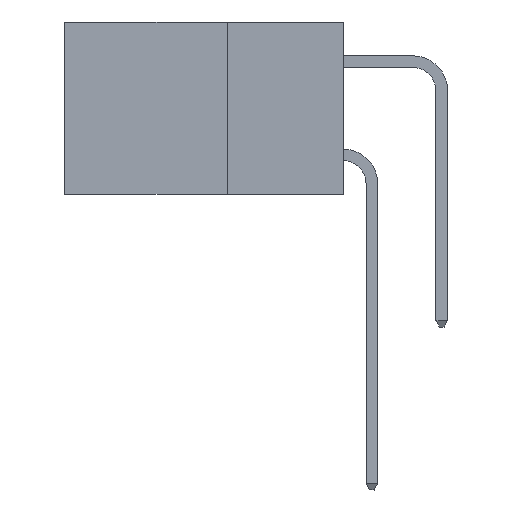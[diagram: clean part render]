
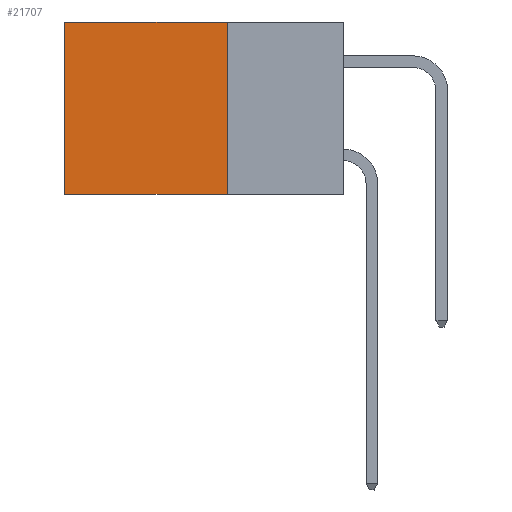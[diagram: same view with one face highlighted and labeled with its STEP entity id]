
A CAD part, left-side view. The second image highlights one B-rep face of the part: STEP entity #21707.
In plain terms, the highlighted planar face has unit normal (-1, 0, 0).
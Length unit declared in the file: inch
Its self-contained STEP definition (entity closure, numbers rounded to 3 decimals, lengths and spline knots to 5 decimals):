
#873 = LINE ( 'NONE', #14879, #6873 ) ;
#923 = ORIENTED_EDGE ( 'NONE', *, *, #19114, .T. ) ;
#928 = CARTESIAN_POINT ( 'NONE',  ( 0.2615, 0.25, -0.37 ) ) ;
#1483 = CARTESIAN_POINT ( 'NONE',  ( 0.2615, 0.25, 0. ) ) ;
#2189 = CARTESIAN_POINT ( 'NONE',  ( 0.2615, 0.25, -0.37 ) ) ;
#2313 = AXIS2_PLACEMENT_3D ( 'NONE', #5311, #12302, #3360 ) ;
#2867 = VECTOR ( 'NONE', #5848, 39.37008 ) ;
#2991 = VERTEX_POINT ( 'NONE', #1483 ) ;
#3360 = DIRECTION ( 'NONE',  ( 0., 0., -1. ) ) ;
#3834 = ORIENTED_EDGE ( 'NONE', *, *, #14002, .T. ) ;
#3910 = LINE ( 'NONE', #2189, #2867 ) ;
#4066 = VECTOR ( 'NONE', #19971, 39.37008 ) ;
#4170 = LINE ( 'NONE', #14845, #10130 ) ;
#4768 = ORIENTED_EDGE ( 'NONE', *, *, #12887, .F. ) ;
#5311 = CARTESIAN_POINT ( 'NONE',  ( 0.2615, 0.25, -0.37 ) ) ;
#5848 = DIRECTION ( 'NONE',  ( 0., 1., 0. ) ) ;
#6873 = VECTOR ( 'NONE', #21893, 39.37008 ) ;
#6913 = FACE_OUTER_BOUND ( 'NONE', #11136, .T. ) ;
#10130 = VECTOR ( 'NONE', #16350, 39.37008 ) ;
#11136 = EDGE_LOOP ( 'NONE', ( #923, #19903, #4768, #3834 ) ) ;
#11342 = CARTESIAN_POINT ( 'NONE',  ( 0.2615, 0.6, -0.37 ) ) ;
#11467 = LINE ( 'NONE', #11342, #4066 ) ;
#12302 = DIRECTION ( 'NONE',  ( 1., 0., 0. ) ) ;
#12887 = EDGE_CURVE ( 'NONE', #2991, #14870, #4170, .T. ) ;
#13918 = PLANE ( 'NONE',  #2313 ) ;
#14002 = EDGE_CURVE ( 'NONE', #2991, #18665, #873, .T. ) ;
#14845 = CARTESIAN_POINT ( 'NONE',  ( 0.2615, 0.25, -0.37 ) ) ;
#14870 = VERTEX_POINT ( 'NONE', #928 ) ;
#14879 = CARTESIAN_POINT ( 'NONE',  ( 0.2615, 0.25, 0. ) ) ;
#15272 = EDGE_CURVE ( 'NONE', #14870, #18851, #3910, .T. ) ;
#15301 = CARTESIAN_POINT ( 'NONE',  ( 0.2615, 0.6, -0.37 ) ) ;
#16350 = DIRECTION ( 'NONE',  ( 0., 0., -1. ) ) ;
#18665 = VERTEX_POINT ( 'NONE', #19996 ) ;
#18851 = VERTEX_POINT ( 'NONE', #15301 ) ;
#19114 = EDGE_CURVE ( 'NONE', #18665, #18851, #11467, .T. ) ;
#19903 = ORIENTED_EDGE ( 'NONE', *, *, #15272, .F. ) ;
#19971 = DIRECTION ( 'NONE',  ( 0., 0., -1. ) ) ;
#19996 = CARTESIAN_POINT ( 'NONE',  ( 0.2615, 0.6, 0. ) ) ;
#21707 = ADVANCED_FACE ( 'NONE', ( #6913 ), #13918, .F. ) ;
#21893 = DIRECTION ( 'NONE',  ( 0., 1., 0. ) ) ;
